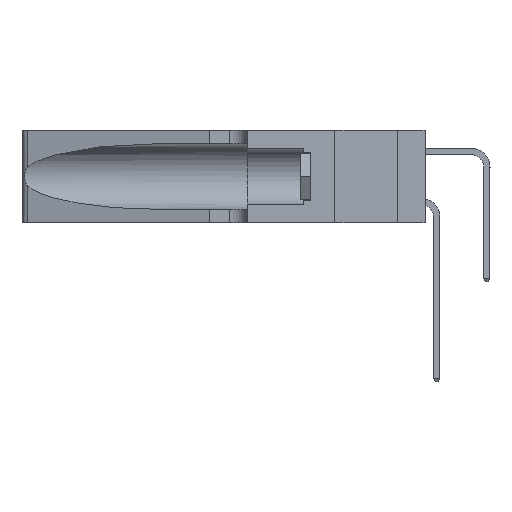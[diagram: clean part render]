
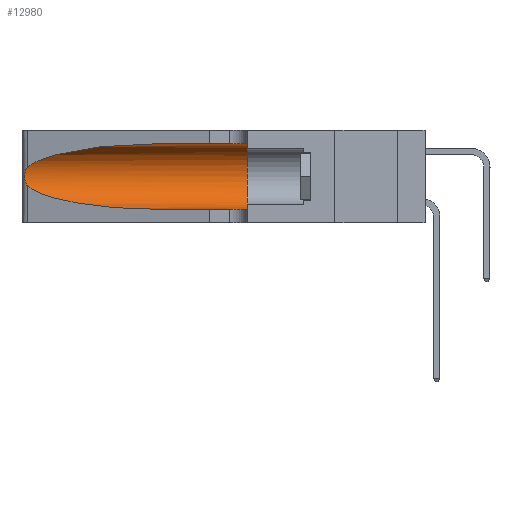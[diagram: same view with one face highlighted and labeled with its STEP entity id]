
A CAD part, left-side view. The second image highlights one B-rep face of the part: STEP entity #12980.
In plain terms, the highlighted cylindrical face has radius 3.308 mm (diameter 6.617 mm), a partial arc.
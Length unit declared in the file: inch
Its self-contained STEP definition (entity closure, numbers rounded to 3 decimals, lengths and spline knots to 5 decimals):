
#1030 = CARTESIAN_POINT ( 'NONE',  ( 0.25555, 1.22994, 0.2215 ) ) ;
#1068 = DIRECTION ( 'NONE',  ( 0., 0., 1. ) ) ;
#1140 = CARTESIAN_POINT ( 'NONE',  ( 0.26018, 1.23835, 0.19895 ) ) ;
#1201 = AXIS2_PLACEMENT_3D ( 'NONE', #29439, #27105, #15390 ) ;
#1252 = CARTESIAN_POINT ( 'NONE',  ( 0.2373, 1.15595, 0.08982 ) ) ;
#1461 = ORIENTED_EDGE ( 'NONE', *, *, #25785, .T. ) ;
#2372 = VERTEX_POINT ( 'NONE', #9923 ) ;
#2498 = EDGE_CURVE ( 'NONE', #13666, #2372, #27454, .T. ) ;
#2840 =( BOUNDED_CURVE ( )  B_SPLINE_CURVE ( 3, ( #7531, #17108, #10020, #26545 ),
 .UNSPECIFIED., .F., .F. ) 
 B_SPLINE_CURVE_WITH_KNOTS ( ( 4, 4 ),
 ( 1.5708, 2.84003 ),
 .UNSPECIFIED. ) 
 CURVE ( )  GEOMETRIC_REPRESENTATION_ITEM ( )  RATIONAL_B_SPLINE_CURVE ( ( 1., 0.87, 0.87, 1. ) ) 
 REPRESENTATION_ITEM ( '' )  );
#3023 = ORIENTED_EDGE ( 'NONE', *, *, #20959, .T. ) ;
#3044 = CARTESIAN_POINT ( 'NONE',  ( 0.1305, 1.61858, 0.05475 ) ) ;
#3670 = CARTESIAN_POINT ( 'NONE',  ( 0.26075, 1.23896, 0.178 ) ) ;
#3729 = B_SPLINE_CURVE_WITH_KNOTS ( 'NONE', 3,
 ( #22837, #1030, #13451, #29861, #15815, #1140, #18186, #3670, #20562, #6233, #22938, #8656, #25294, #11145 ),
 .UNSPECIFIED., .F., .F.,
 ( 4, 2, 2, 2, 2, 2, 4 ),
 ( 0., 0.00027, 0.00053, 0.00107, 0.0016, 0.00187, 0.00214 ),
 .UNSPECIFIED. ) ;
#4534 = VERTEX_POINT ( 'NONE', #23307 ) ;
#4998 = VERTEX_POINT ( 'NONE', #9075 ) ;
#6219 =( BOUNDED_CURVE ( )  B_SPLINE_CURVE ( 3, ( #18310, #1252, #6352, #23055 ),
 .UNSPECIFIED., .F., .F. ) 
 B_SPLINE_CURVE_WITH_KNOTS ( ( 4, 4 ),
 ( 3.44316, 4.71239 ),
 .UNSPECIFIED. ) 
 CURVE ( )  GEOMETRIC_REPRESENTATION_ITEM ( )  RATIONAL_B_SPLINE_CURVE ( ( 1., 0.87, 0.87, 1. ) ) 
 REPRESENTATION_ITEM ( '' )  );
#6233 = CARTESIAN_POINT ( 'NONE',  ( 0.25856, 1.23593, 0.16098 ) ) ;
#6352 = CARTESIAN_POINT ( 'NONE',  ( 0.18966, 0.96281, 0.05475 ) ) ;
#6391 = VERTEX_POINT ( 'NONE', #30177 ) ;
#7368 = VERTEX_POINT ( 'NONE', #17223 ) ;
#7531 = CARTESIAN_POINT ( 'NONE',  ( 0.1305, 0.72297, 0.31525 ) ) ;
#8656 = CARTESIAN_POINT ( 'NONE',  ( 0.25639, 1.23186, 0.15144 ) ) ;
#9075 = CARTESIAN_POINT ( 'NONE',  ( 0.25487, 1.22718, 0.22369 ) ) ;
#9594 = CARTESIAN_POINT ( 'NONE',  ( 0.1305, 1.61858, 0.31525 ) ) ;
#9923 = CARTESIAN_POINT ( 'NONE',  ( 0.1305, 0.35, 0.05475 ) ) ;
#10020 = CARTESIAN_POINT ( 'NONE',  ( 0.2373, 1.15595, 0.28018 ) ) ;
#10582 = EDGE_CURVE ( 'NONE', #7368, #13666, #6219, .T. ) ;
#11145 = CARTESIAN_POINT ( 'NONE',  ( 0.25487, 1.22718, 0.14631 ) ) ;
#12817 = LINE ( 'NONE', #9594, #30072 ) ;
#12980 = ADVANCED_FACE ( 'NONE', ( #13296 ), #30537, .F. ) ;
#13296 = FACE_OUTER_BOUND ( 'NONE', #21436, .T. ) ;
#13451 = CARTESIAN_POINT ( 'NONE',  ( 0.25639, 1.23184, 0.21858 ) ) ;
#13666 = VERTEX_POINT ( 'NONE', #28716 ) ;
#15390 = DIRECTION ( 'NONE',  ( 0., 0., -1. ) ) ;
#15739 = DIRECTION ( 'NONE',  ( 0., 1., 0. ) ) ;
#15815 = CARTESIAN_POINT ( 'NONE',  ( 0.25854, 1.2359, 0.20912 ) ) ;
#16020 = ORIENTED_EDGE ( 'NONE', *, *, #10582, .T. ) ;
#17108 = CARTESIAN_POINT ( 'NONE',  ( 0.18966, 0.96281, 0.31525 ) ) ;
#17223 = CARTESIAN_POINT ( 'NONE',  ( 0.25487, 1.22718, 0.14631 ) ) ;
#17521 = ORIENTED_EDGE ( 'NONE', *, *, #2498, .T. ) ;
#17829 = ORIENTED_EDGE ( 'NONE', *, *, #19958, .F. ) ;
#18186 = CARTESIAN_POINT ( 'NONE',  ( 0.26075, 1.23896, 0.19203 ) ) ;
#18310 = CARTESIAN_POINT ( 'NONE',  ( 0.25487, 1.22718, 0.14631 ) ) ;
#19630 = AXIS2_PLACEMENT_3D ( 'NONE', #29794, #15739, #1068 ) ;
#19958 = EDGE_CURVE ( 'NONE', #4534, #6391, #12817, .T. ) ;
#19987 = DIRECTION ( 'NONE',  ( 0., -1., 0. ) ) ;
#20562 = CARTESIAN_POINT ( 'NONE',  ( 0.26017, 1.23833, 0.17102 ) ) ;
#20959 = EDGE_CURVE ( 'NONE', #4998, #7368, #3729, .T. ) ;
#21436 = EDGE_LOOP ( 'NONE', ( #1461, #3023, #16020, #17521, #23777, #17829 ) ) ;
#21982 = VECTOR ( 'NONE', #19987, 39.37008 ) ;
#22837 = CARTESIAN_POINT ( 'NONE',  ( 0.25487, 1.22718, 0.22369 ) ) ;
#22938 = CARTESIAN_POINT ( 'NONE',  ( 0.25789, 1.23486, 0.15765 ) ) ;
#23055 = CARTESIAN_POINT ( 'NONE',  ( 0.1305, 0.72297, 0.05475 ) ) ;
#23307 = CARTESIAN_POINT ( 'NONE',  ( 0.1305, 0.72297, 0.31525 ) ) ;
#23666 = CIRCLE ( 'NONE', #19630, 0.13025 ) ;
#23777 = ORIENTED_EDGE ( 'NONE', *, *, #29981, .F. ) ;
#25294 = CARTESIAN_POINT ( 'NONE',  ( 0.25555, 1.22993, 0.14849 ) ) ;
#25785 = EDGE_CURVE ( 'NONE', #4534, #4998, #2840, .T. ) ;
#26545 = CARTESIAN_POINT ( 'NONE',  ( 0.25487, 1.22718, 0.22369 ) ) ;
#27105 = DIRECTION ( 'NONE',  ( 0., -1., 0. ) ) ;
#27454 = LINE ( 'NONE', #3044, #21982 ) ;
#28490 = DIRECTION ( 'NONE',  ( 0., -1., 0. ) ) ;
#28716 = CARTESIAN_POINT ( 'NONE',  ( 0.1305, 0.72297, 0.05475 ) ) ;
#29439 = CARTESIAN_POINT ( 'NONE',  ( 0.1305, 1.61858, 0.185 ) ) ;
#29794 = CARTESIAN_POINT ( 'NONE',  ( 0.1305, 0.35, 0.185 ) ) ;
#29861 = CARTESIAN_POINT ( 'NONE',  ( 0.25787, 1.23484, 0.2124 ) ) ;
#29981 = EDGE_CURVE ( 'NONE', #6391, #2372, #23666, .T. ) ;
#30072 = VECTOR ( 'NONE', #28490, 39.37008 ) ;
#30177 = CARTESIAN_POINT ( 'NONE',  ( 0.1305, 0.35, 0.31525 ) ) ;
#30537 = CYLINDRICAL_SURFACE ( 'NONE', #1201, 0.13025 ) ;
